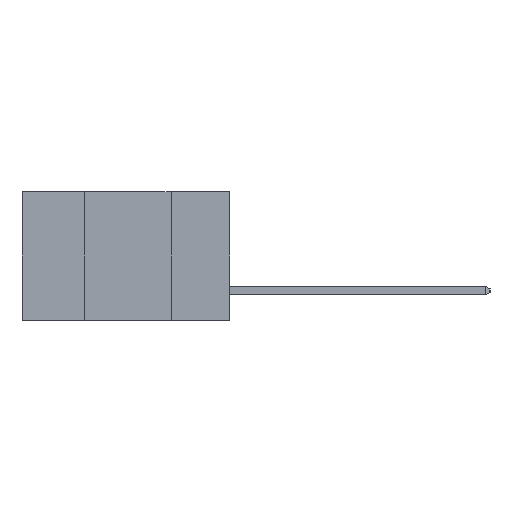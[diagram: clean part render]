
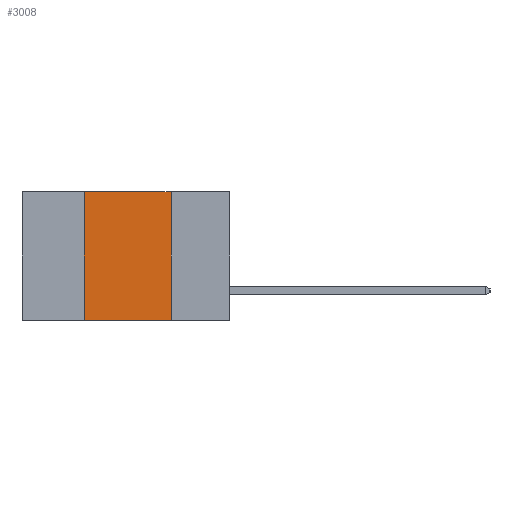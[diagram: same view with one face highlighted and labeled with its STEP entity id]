
A CAD part, left-side view. The second image highlights one B-rep face of the part: STEP entity #3008.
In plain terms, the highlighted planar face has unit normal (-1, 0, 0).
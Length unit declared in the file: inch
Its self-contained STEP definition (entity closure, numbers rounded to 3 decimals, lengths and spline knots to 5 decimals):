
#165 = CARTESIAN_POINT ( 'NONE',  ( 0., 0.17, 0. ) ) ;
#630 = CARTESIAN_POINT ( 'NONE',  ( 0., 0.6, 0. ) ) ;
#1291 = VERTEX_POINT ( 'NONE', #10822 ) ;
#1776 = CARTESIAN_POINT ( 'NONE',  ( 0., 0.17, -0.37 ) ) ;
#1777 = FACE_OUTER_BOUND ( 'NONE', #10691, .T. ) ;
#1892 = DIRECTION ( 'NONE',  ( 1., 0., 0. ) ) ;
#3008 = ADVANCED_FACE ( 'NONE', ( #1777 ), #12313, .F. ) ;
#3111 = VERTEX_POINT ( 'NONE', #1776 ) ;
#3311 = DIRECTION ( 'NONE',  ( 0., -1., 0. ) ) ;
#4423 = LINE ( 'NONE', #165, #10585 ) ;
#4590 = EDGE_CURVE ( 'NONE', #1291, #3111, #4423, .T. ) ;
#4956 = AXIS2_PLACEMENT_3D ( 'NONE', #630, #1892, #5070 ) ;
#5070 = DIRECTION ( 'NONE',  ( 0., 0., -1. ) ) ;
#5356 = VECTOR ( 'NONE', #12324, 39.37008 ) ;
#6344 = ORIENTED_EDGE ( 'NONE', *, *, #8541, .F. ) ;
#6684 = ORIENTED_EDGE ( 'NONE', *, *, #11089, .F. ) ;
#7190 = CARTESIAN_POINT ( 'NONE',  ( 0., 0.6, -0.37 ) ) ;
#7269 = CARTESIAN_POINT ( 'NONE',  ( 0., 0.42, 0. ) ) ;
#7582 = LINE ( 'NONE', #13029, #13227 ) ;
#7726 = DIRECTION ( 'NONE',  ( 0., 0., 1. ) ) ;
#7788 = VECTOR ( 'NONE', #3311, 39.37008 ) ;
#8541 = EDGE_CURVE ( 'NONE', #13718, #1291, #13448, .T. ) ;
#9345 = VERTEX_POINT ( 'NONE', #10476 ) ;
#9409 = EDGE_CURVE ( 'NONE', #9345, #3111, #13614, .T. ) ;
#9621 = ORIENTED_EDGE ( 'NONE', *, *, #9409, .T. ) ;
#10476 = CARTESIAN_POINT ( 'NONE',  ( 0., 0.42, -0.37 ) ) ;
#10569 = CARTESIAN_POINT ( 'NONE',  ( 0., 0.6, 0. ) ) ;
#10585 = VECTOR ( 'NONE', #10870, 39.37008 ) ;
#10691 = EDGE_LOOP ( 'NONE', ( #11774, #6344, #6684, #9621 ) ) ;
#10822 = CARTESIAN_POINT ( 'NONE',  ( 0., 0.17, 0. ) ) ;
#10870 = DIRECTION ( 'NONE',  ( 0., 0., -1. ) ) ;
#11089 = EDGE_CURVE ( 'NONE', #9345, #13718, #7582, .T. ) ;
#11774 = ORIENTED_EDGE ( 'NONE', *, *, #4590, .F. ) ;
#12313 = PLANE ( 'NONE',  #4956 ) ;
#12324 = DIRECTION ( 'NONE',  ( 0., -1., 0. ) ) ;
#13029 = CARTESIAN_POINT ( 'NONE',  ( 0., 0.42, 0. ) ) ;
#13227 = VECTOR ( 'NONE', #7726, 39.37008 ) ;
#13448 = LINE ( 'NONE', #10569, #7788 ) ;
#13614 = LINE ( 'NONE', #7190, #5356 ) ;
#13718 = VERTEX_POINT ( 'NONE', #7269 ) ;
